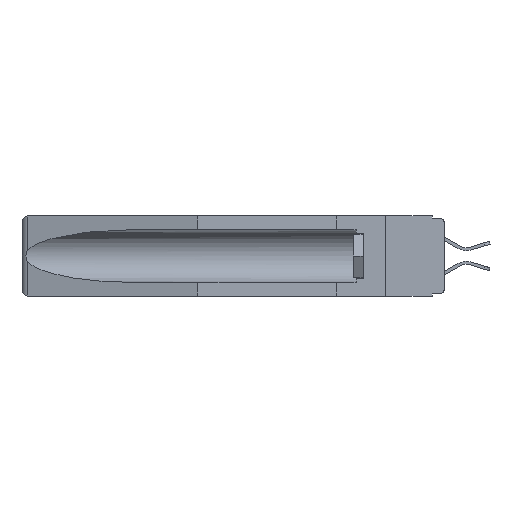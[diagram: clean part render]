
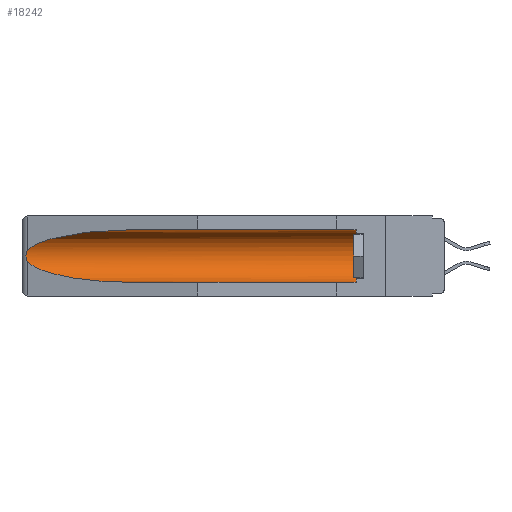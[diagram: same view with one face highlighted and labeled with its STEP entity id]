
A CAD part, left-side view. The second image highlights one B-rep face of the part: STEP entity #18242.
In plain terms, the highlighted cylindrical face has radius 2.857 mm (diameter 5.715 mm), a partial arc.
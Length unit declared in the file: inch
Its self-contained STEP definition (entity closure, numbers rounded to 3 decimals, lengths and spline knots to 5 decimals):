
#207 = VERTEX_POINT ( 'NONE', #10522 ) ;
#566 = VERTEX_POINT ( 'NONE', #23169 ) ;
#755 = CARTESIAN_POINT ( 'NONE',  ( 0.155, 1.07973, -0.284 ) ) ;
#770 = DIRECTION ( 'NONE',  ( 0., 0., 1. ) ) ;
#1179 = CARTESIAN_POINT ( 'NONE',  ( 0.25451, 1.48313, -0.09465 ) ) ;
#1196 = CARTESIAN_POINT ( 'NONE',  ( 0.155, -0.30754, -0.059 ) ) ;
#2448 = DIRECTION ( 'NONE',  ( 0., 1., 0. ) ) ;
#3273 = CARTESIAN_POINT ( 'NONE',  ( 0.26654, 1.53092, -0.15636 ) ) ;
#3281 = CARTESIAN_POINT ( 'NONE',  ( 0.155, -0.30754, -0.1715 ) ) ;
#3365 = DIRECTION ( 'NONE',  ( 0., 1., 0. ) ) ;
#3980 = EDGE_CURVE ( 'NONE', #207, #5591, #23455, .T. ) ;
#4401 = DIRECTION ( 'NONE',  ( 0., -1., 0. ) ) ;
#5591 = VERTEX_POINT ( 'NONE', #14761 ) ;
#6215 = CARTESIAN_POINT ( 'NONE',  ( 0.155, 0.126, -0.1715 ) ) ;
#6714 = EDGE_CURVE ( 'NONE', #207, #15977, #20838, .T. ) ;
#6823 = CARTESIAN_POINT ( 'NONE',  ( 0.26537, 1.52718, -0.14972 ) ) ;
#7001 = CARTESIAN_POINT ( 'NONE',  ( 0.2673, 1.5327, -0.16383 ) ) ;
#7106 = CARTESIAN_POINT ( 'NONE',  ( 0.2673, 1.53269, -0.17917 ) ) ;
#7410 = ORIENTED_EDGE ( 'NONE', *, *, #19949, .T. ) ;
#7932 = VECTOR ( 'NONE', #2448, 39.37008 ) ;
#8031 = ORIENTED_EDGE ( 'NONE', *, *, #19558, .T. ) ;
#8321 = FACE_OUTER_BOUND ( 'NONE', #13993, .T. ) ;
#8424 = ORIENTED_EDGE ( 'NONE', *, *, #6714, .F. ) ;
#8451 = CYLINDRICAL_SURFACE ( 'NONE', #23173, 0.1125 ) ;
#8563 = DIRECTION ( 'NONE',  ( 0., 0., 1. ) ) ;
#8822 = CARTESIAN_POINT ( 'NONE',  ( 0.155, 1.07973, -0.059 ) ) ;
#8910 = CARTESIAN_POINT ( 'NONE',  ( 0.2675, 1.53308, -0.17534 ) ) ;
#9624 =( BOUNDED_CURVE ( )  B_SPLINE_CURVE ( 3, ( #23385, #23738, #1179, #6823 ),
 .UNSPECIFIED., .F., .F. ) 
 B_SPLINE_CURVE_WITH_KNOTS ( ( 4, 4 ),
 ( 4.71239, 6.08839 ),
 .UNSPECIFIED. ) 
 CURVE ( )  GEOMETRIC_REPRESENTATION_ITEM ( )  RATIONAL_B_SPLINE_CURVE ( ( 1., 0.848, 0.848, 1. ) ) 
 REPRESENTATION_ITEM ( '' )  );
#10014 = B_SPLINE_CURVE_WITH_KNOTS ( 'NONE', 3,
 ( #20060, #16278, #3273, #7001, #10393, #8910, #7106, #14475, #12313, #12544 ),
 .UNSPECIFIED., .F., .F.,
 ( 4, 2, 2, 2, 4 ),
 ( 0., 0.00029, 0.00058, 0.00087, 0.00117 ),
 .UNSPECIFIED. ) ;
#10393 = CARTESIAN_POINT ( 'NONE',  ( 0.2675, 1.53308, -0.16763 ) ) ;
#10404 = DIRECTION ( 'NONE',  ( 0., 1., 0. ) ) ;
#10522 = CARTESIAN_POINT ( 'NONE',  ( 0.155, 0.126, -0.284 ) ) ;
#11069 = CARTESIAN_POINT ( 'NONE',  ( 0.26537, 1.52718, -0.14972 ) ) ;
#12313 = CARTESIAN_POINT ( 'NONE',  ( 0.26597, 1.5296, -0.19026 ) ) ;
#12544 = CARTESIAN_POINT ( 'NONE',  ( 0.26537, 1.52718, -0.19328 ) ) ;
#13802 = AXIS2_PLACEMENT_3D ( 'NONE', #6215, #4401, #770 ) ;
#13993 = EDGE_LOOP ( 'NONE', ( #18450, #8031, #17056, #8424, #17744, #7410 ) ) ;
#14210 = LINE ( 'NONE', #1196, #18877 ) ;
#14475 = CARTESIAN_POINT ( 'NONE',  ( 0.26655, 1.53094, -0.18657 ) ) ;
#14761 = CARTESIAN_POINT ( 'NONE',  ( 0.155, 0.126, -0.059 ) ) ;
#15977 = VERTEX_POINT ( 'NONE', #22678 ) ;
#16088 =( BOUNDED_CURVE ( )  B_SPLINE_CURVE ( 3, ( #18986, #17130, #20586, #755 ),
 .UNSPECIFIED., .F., .F. ) 
 B_SPLINE_CURVE_WITH_KNOTS ( ( 4, 4 ),
 ( 0.1948, 1.5708 ),
 .UNSPECIFIED. ) 
 CURVE ( )  GEOMETRIC_REPRESENTATION_ITEM ( )  RATIONAL_B_SPLINE_CURVE ( ( 1., 0.848, 0.848, 1. ) ) 
 REPRESENTATION_ITEM ( '' )  );
#16278 = CARTESIAN_POINT ( 'NONE',  ( 0.26597, 1.52961, -0.15275 ) ) ;
#17056 = ORIENTED_EDGE ( 'NONE', *, *, #18192, .T. ) ;
#17130 = CARTESIAN_POINT ( 'NONE',  ( 0.25451, 1.48313, -0.24835 ) ) ;
#17744 = ORIENTED_EDGE ( 'NONE', *, *, #3980, .T. ) ;
#18192 = EDGE_CURVE ( 'NONE', #566, #15977, #16088, .T. ) ;
#18242 = ADVANCED_FACE ( 'NONE', ( #8321 ), #8451, .F. ) ;
#18450 = ORIENTED_EDGE ( 'NONE', *, *, #23828, .T. ) ;
#18510 = CARTESIAN_POINT ( 'NONE',  ( 0.155, -0.30754, -0.284 ) ) ;
#18723 = VERTEX_POINT ( 'NONE', #11069 ) ;
#18877 = VECTOR ( 'NONE', #3365, 39.37008 ) ;
#18986 = CARTESIAN_POINT ( 'NONE',  ( 0.26537, 1.52718, -0.19328 ) ) ;
#19558 = EDGE_CURVE ( 'NONE', #18723, #566, #10014, .T. ) ;
#19949 = EDGE_CURVE ( 'NONE', #5591, #20545, #14210, .T. ) ;
#20060 = CARTESIAN_POINT ( 'NONE',  ( 0.26537, 1.52718, -0.14972 ) ) ;
#20545 = VERTEX_POINT ( 'NONE', #8822 ) ;
#20586 = CARTESIAN_POINT ( 'NONE',  ( 0.21114, 1.30732, -0.284 ) ) ;
#20838 = LINE ( 'NONE', #18510, #7932 ) ;
#22678 = CARTESIAN_POINT ( 'NONE',  ( 0.155, 1.07973, -0.284 ) ) ;
#23169 = CARTESIAN_POINT ( 'NONE',  ( 0.26537, 1.52718, -0.19328 ) ) ;
#23173 = AXIS2_PLACEMENT_3D ( 'NONE', #3281, #10404, #8563 ) ;
#23385 = CARTESIAN_POINT ( 'NONE',  ( 0.155, 1.07973, -0.059 ) ) ;
#23455 = CIRCLE ( 'NONE', #13802, 0.1125 ) ;
#23738 = CARTESIAN_POINT ( 'NONE',  ( 0.21114, 1.30732, -0.059 ) ) ;
#23828 = EDGE_CURVE ( 'NONE', #20545, #18723, #9624, .T. ) ;
